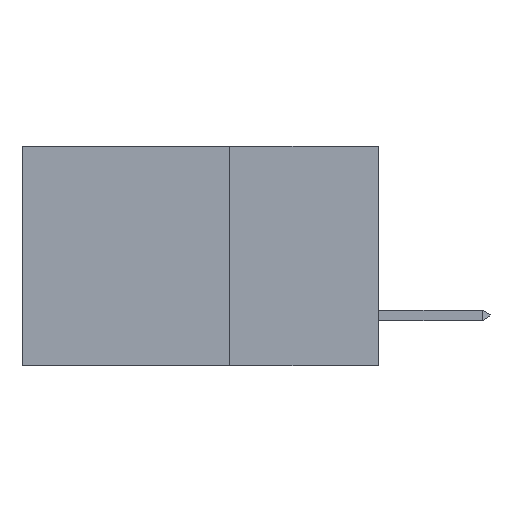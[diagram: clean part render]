
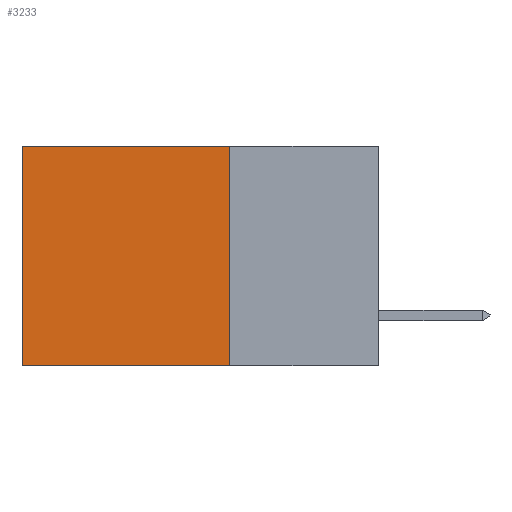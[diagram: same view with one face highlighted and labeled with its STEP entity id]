
A CAD part, left-side view. The second image highlights one B-rep face of the part: STEP entity #3233.
In plain terms, the highlighted planar face has unit normal (-1, 0, 0).
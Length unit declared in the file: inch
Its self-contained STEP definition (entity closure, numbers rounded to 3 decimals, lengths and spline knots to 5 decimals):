
#24 = CARTESIAN_POINT ( 'NONE',  ( 0.298, 0.6, 0. ) ) ;
#214 = DIRECTION ( 'NONE',  ( 0., 0., -1. ) ) ;
#512 = DIRECTION ( 'NONE',  ( 0., 1., 0. ) ) ;
#605 = CARTESIAN_POINT ( 'NONE',  ( 0.298, 0.25, -0.37 ) ) ;
#826 = VERTEX_POINT ( 'NONE', #24 ) ;
#1271 = VERTEX_POINT ( 'NONE', #8125 ) ;
#1383 = EDGE_LOOP ( 'NONE', ( #6900, #7143, #9322, #5321 ) ) ;
#1621 = CARTESIAN_POINT ( 'NONE',  ( 0.298, 0.25, 0. ) ) ;
#1724 = CARTESIAN_POINT ( 'NONE',  ( 0.298, 0.25, 0. ) ) ;
#2799 = LINE ( 'NONE', #7982, #6828 ) ;
#2980 = FACE_OUTER_BOUND ( 'NONE', #1383, .T. ) ;
#3233 = ADVANCED_FACE ( 'NONE', ( #2980 ), #5329, .F. ) ;
#4097 = CARTESIAN_POINT ( 'NONE',  ( 0.298, 0.25, 0. ) ) ;
#5197 = EDGE_CURVE ( 'NONE', #8716, #826, #8999, .T. ) ;
#5321 = ORIENTED_EDGE ( 'NONE', *, *, #5197, .T. ) ;
#5329 = PLANE ( 'NONE',  #8286 ) ;
#5491 = DIRECTION ( 'NONE',  ( 1., 0., 0. ) ) ;
#5586 = DIRECTION ( 'NONE',  ( 0., 1., 0. ) ) ;
#5708 = LINE ( 'NONE', #10162, #6813 ) ;
#6071 = EDGE_CURVE ( 'NONE', #826, #1271, #2799, .T. ) ;
#6813 = VECTOR ( 'NONE', #512, 39.37008 ) ;
#6828 = VECTOR ( 'NONE', #7157, 39.37008 ) ;
#6845 = VECTOR ( 'NONE', #5586, 39.37008 ) ;
#6900 = ORIENTED_EDGE ( 'NONE', *, *, #6071, .T. ) ;
#7143 = ORIENTED_EDGE ( 'NONE', *, *, #7442, .F. ) ;
#7157 = DIRECTION ( 'NONE',  ( 0., 0., -1. ) ) ;
#7197 = DIRECTION ( 'NONE',  ( 0., 0., -1. ) ) ;
#7442 = EDGE_CURVE ( 'NONE', #9129, #1271, #5708, .T. ) ;
#7982 = CARTESIAN_POINT ( 'NONE',  ( 0.298, 0.6, 0. ) ) ;
#8047 = VECTOR ( 'NONE', #7197, 39.37008 ) ;
#8125 = CARTESIAN_POINT ( 'NONE',  ( 0.298, 0.6, -0.37 ) ) ;
#8286 = AXIS2_PLACEMENT_3D ( 'NONE', #1724, #5491, #214 ) ;
#8623 = EDGE_CURVE ( 'NONE', #8716, #9129, #9968, .T. ) ;
#8716 = VERTEX_POINT ( 'NONE', #4097 ) ;
#8999 = LINE ( 'NONE', #10307, #6845 ) ;
#9129 = VERTEX_POINT ( 'NONE', #605 ) ;
#9322 = ORIENTED_EDGE ( 'NONE', *, *, #8623, .F. ) ;
#9968 = LINE ( 'NONE', #1621, #8047 ) ;
#10162 = CARTESIAN_POINT ( 'NONE',  ( 0.298, 0.25, -0.37 ) ) ;
#10307 = CARTESIAN_POINT ( 'NONE',  ( 0.298, 0.25, 0. ) ) ;
